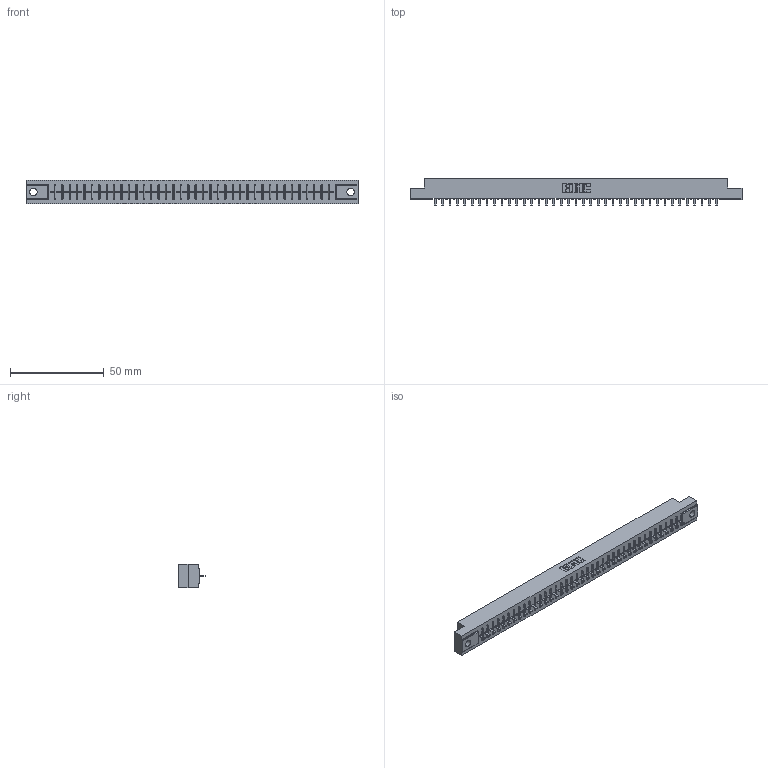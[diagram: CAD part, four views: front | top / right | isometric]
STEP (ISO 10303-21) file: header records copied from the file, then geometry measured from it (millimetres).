
FILE_DESCRIPTION (( 'STEP AP203' ), '1' );
FILE_NAME ('306-039-521-104.STEP', '2019-09-12T00:14:23', ( '' ), ( '' ), 'SwSTEP 2.0', 'SolidWorks 2016', '' );
FILE_SCHEMA (( 'CONFIG_CONTROL_DESIGN' ));
Length unit declared in the file: inch
Products named in the file (3): 306-290-001_121; 306 Part_.156 Dia; 306-039-521-104
Assembly tree (40 placements, depth 2):
  306-039-521-104
    306 Part_.156 Dia
    306-290-001_121  x39
Bounding box: 177.55 x 14.88 x 12.7 mm (x, y, z)
Volume: 19450.6 mm3; surface area: 19467.1 mm2
Topology: 40 solids, 40 shells, 2860 faces, 8035 edges, 5146 vertices
Faces by surface type: plane 1915, cylinder 789, sphere 156
Entity records: 37132 total; most frequent: CARTESIAN_POINT 6238, ORIENTED_EDGE 6182, DIRECTION 6143, EDGE_CURVE 3091, LINE 2425, VECTOR 2425, VERTEX_POINT 1954, AXIS2_PLACEMENT_3D 1859
